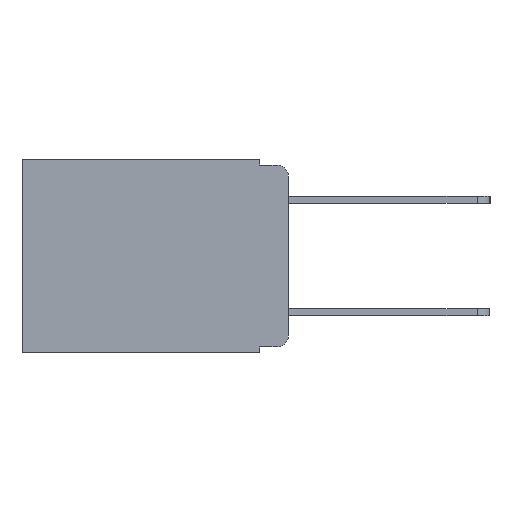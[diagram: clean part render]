
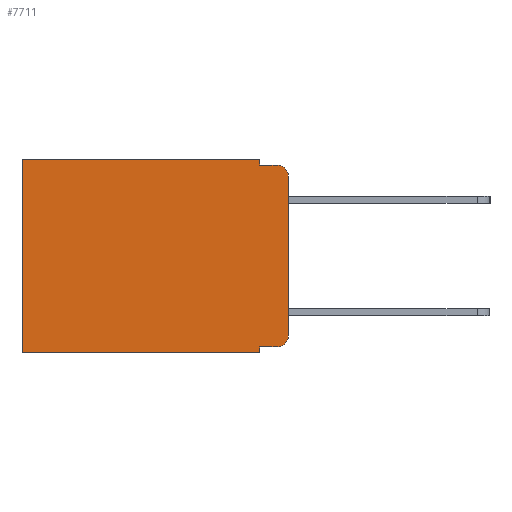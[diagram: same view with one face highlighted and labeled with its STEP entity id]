
A CAD part, left-side view. The second image highlights one B-rep face of the part: STEP entity #7711.
In plain terms, the highlighted planar face has unit normal (-1, 0, 0).
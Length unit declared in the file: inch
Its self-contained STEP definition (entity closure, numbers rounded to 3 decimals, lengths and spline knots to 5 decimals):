
#279 = DIRECTION ( 'NONE',  ( 0., -1., 0. ) ) ;
#445 = ORIENTED_EDGE ( 'NONE', *, *, #1845, .T. ) ;
#650 = ORIENTED_EDGE ( 'NONE', *, *, #10592, .F. ) ;
#675 = DIRECTION ( 'NONE',  ( 0., 0., -1. ) ) ;
#715 = CARTESIAN_POINT ( 'NONE',  ( 0.298, 0.02, -0.313 ) ) ;
#947 = CARTESIAN_POINT ( 'NONE',  ( 0.298, 0.051, 0. ) ) ;
#1322 = CARTESIAN_POINT ( 'NONE',  ( 0.298, 0.051, -0.333 ) ) ;
#1445 = DIRECTION ( 'NONE',  ( 0., 1., 0. ) ) ;
#1460 = DIRECTION ( 'NONE',  ( -1., 0., 0. ) ) ;
#1650 = CARTESIAN_POINT ( 'NONE',  ( 0.298, 0., 0. ) ) ;
#1845 = EDGE_CURVE ( 'NONE', #9533, #2233, #6009, .T. ) ;
#2096 = CARTESIAN_POINT ( 'NONE',  ( 0.298, 0.473, 0. ) ) ;
#2152 = PLANE ( 'NONE',  #11686 ) ;
#2233 = VERTEX_POINT ( 'NONE', #8018 ) ;
#2417 = DIRECTION ( 'NONE',  ( -1., 0., 0. ) ) ;
#2543 = VECTOR ( 'NONE', #2950, 39.37008 ) ;
#2566 = EDGE_LOOP ( 'NONE', ( #650, #5002, #6541, #6428, #7224, #11997, #8899, #5965, #5887, #445 ) ) ;
#2593 = EDGE_CURVE ( 'NONE', #10687, #7133, #12254, .T. ) ;
#2950 = DIRECTION ( 'NONE',  ( 0., 0., -1. ) ) ;
#2981 = LINE ( 'NONE', #2096, #8307 ) ;
#3244 = EDGE_CURVE ( 'NONE', #12020, #9160, #4935, .T. ) ;
#4596 = CARTESIAN_POINT ( 'NONE',  ( 0.298, 0.02, -0.333 ) ) ;
#4601 = DIRECTION ( 'NONE',  ( 0., 0., -1. ) ) ;
#4935 = LINE ( 'NONE', #5227, #7904 ) ;
#5002 = ORIENTED_EDGE ( 'NONE', *, *, #8436, .T. ) ;
#5125 = CIRCLE ( 'NONE', #14164, 0.02 ) ;
#5227 = CARTESIAN_POINT ( 'NONE',  ( 0.298, 0., 0. ) ) ;
#5354 = DIRECTION ( 'NONE',  ( 0., 1., 0. ) ) ;
#5887 = ORIENTED_EDGE ( 'NONE', *, *, #7966, .T. ) ;
#5965 = ORIENTED_EDGE ( 'NONE', *, *, #8718, .F. ) ;
#6004 = VECTOR ( 'NONE', #14226, 39.37008 ) ;
#6009 = CIRCLE ( 'NONE', #8349, 0.02 ) ;
#6214 = EDGE_CURVE ( 'NONE', #13782, #12445, #8459, .T. ) ;
#6428 = ORIENTED_EDGE ( 'NONE', *, *, #11534, .F. ) ;
#6517 = VECTOR ( 'NONE', #7208, 39.37008 ) ;
#6541 = ORIENTED_EDGE ( 'NONE', *, *, #6214, .F. ) ;
#6836 = DIRECTION ( 'NONE',  ( 0., 0., -1. ) ) ;
#7026 = FACE_OUTER_BOUND ( 'NONE', #2566, .T. ) ;
#7133 = VERTEX_POINT ( 'NONE', #12358 ) ;
#7139 = VERTEX_POINT ( 'NONE', #10299 ) ;
#7208 = DIRECTION ( 'NONE',  ( 0., -1., 0. ) ) ;
#7224 = ORIENTED_EDGE ( 'NONE', *, *, #3244, .T. ) ;
#7557 = LINE ( 'NONE', #7712, #10417 ) ;
#7711 = ADVANCED_FACE ( 'NONE', ( #7026 ), #2152, .F. ) ;
#7712 = CARTESIAN_POINT ( 'NONE',  ( 0.298, 0.051, 0. ) ) ;
#7904 = VECTOR ( 'NONE', #5354, 39.37008 ) ;
#7927 = CARTESIAN_POINT ( 'NONE',  ( 0.298, 0.051, 0. ) ) ;
#7966 = EDGE_CURVE ( 'NONE', #7139, #9533, #9408, .T. ) ;
#8018 = CARTESIAN_POINT ( 'NONE',  ( 0.298, 0., -0.313 ) ) ;
#8307 = VECTOR ( 'NONE', #6836, 39.37008 ) ;
#8349 = AXIS2_PLACEMENT_3D ( 'NONE', #715, #2417, #11000 ) ;
#8436 = EDGE_CURVE ( 'NONE', #8660, #12445, #5125, .T. ) ;
#8437 = CARTESIAN_POINT ( 'NONE',  ( 0.298, 0.02, -0.03 ) ) ;
#8459 = LINE ( 'NONE', #8468, #11603 ) ;
#8468 = CARTESIAN_POINT ( 'NONE',  ( 0.298, 0.051, -0.01 ) ) ;
#8660 = VERTEX_POINT ( 'NONE', #10866 ) ;
#8718 = EDGE_CURVE ( 'NONE', #7139, #10687, #7557, .T. ) ;
#8899 = ORIENTED_EDGE ( 'NONE', *, *, #2593, .F. ) ;
#8947 = CARTESIAN_POINT ( 'NONE',  ( 0.298, 0.051, -0.01 ) ) ;
#9160 = VERTEX_POINT ( 'NONE', #11707 ) ;
#9219 = CARTESIAN_POINT ( 'NONE',  ( 0.298, 0., -0.343 ) ) ;
#9408 = LINE ( 'NONE', #1322, #6517 ) ;
#9451 = VECTOR ( 'NONE', #1445, 39.37008 ) ;
#9519 = DIRECTION ( 'NONE',  ( 0., 0., -1. ) ) ;
#9533 = VERTEX_POINT ( 'NONE', #4596 ) ;
#10109 = CARTESIAN_POINT ( 'NONE',  ( 0.298, 0., 0. ) ) ;
#10144 = EDGE_CURVE ( 'NONE', #9160, #7133, #2981, .T. ) ;
#10299 = CARTESIAN_POINT ( 'NONE',  ( 0.298, 0.051, -0.333 ) ) ;
#10417 = VECTOR ( 'NONE', #675, 39.37008 ) ;
#10592 = EDGE_CURVE ( 'NONE', #8660, #2233, #14178, .T. ) ;
#10687 = VERTEX_POINT ( 'NONE', #10800 ) ;
#10800 = CARTESIAN_POINT ( 'NONE',  ( 0.298, 0.051, -0.343 ) ) ;
#10866 = CARTESIAN_POINT ( 'NONE',  ( 0.298, 0., -0.03 ) ) ;
#11000 = DIRECTION ( 'NONE',  ( 0., 0., -1. ) ) ;
#11163 = DIRECTION ( 'NONE',  ( 1., 0., 0. ) ) ;
#11534 = EDGE_CURVE ( 'NONE', #12020, #13782, #14149, .T. ) ;
#11603 = VECTOR ( 'NONE', #279, 39.37008 ) ;
#11686 = AXIS2_PLACEMENT_3D ( 'NONE', #10109, #11163, #4601 ) ;
#11707 = CARTESIAN_POINT ( 'NONE',  ( 0.298, 0.473, 0. ) ) ;
#11997 = ORIENTED_EDGE ( 'NONE', *, *, #10144, .T. ) ;
#12020 = VERTEX_POINT ( 'NONE', #7927 ) ;
#12254 = LINE ( 'NONE', #9219, #9451 ) ;
#12358 = CARTESIAN_POINT ( 'NONE',  ( 0.298, 0.473, -0.343 ) ) ;
#12445 = VERTEX_POINT ( 'NONE', #13085 ) ;
#13085 = CARTESIAN_POINT ( 'NONE',  ( 0.298, 0.02, -0.01 ) ) ;
#13782 = VERTEX_POINT ( 'NONE', #8947 ) ;
#14149 = LINE ( 'NONE', #947, #6004 ) ;
#14164 = AXIS2_PLACEMENT_3D ( 'NONE', #8437, #1460, #9519 ) ;
#14178 = LINE ( 'NONE', #1650, #2543 ) ;
#14226 = DIRECTION ( 'NONE',  ( 0., 0., -1. ) ) ;
